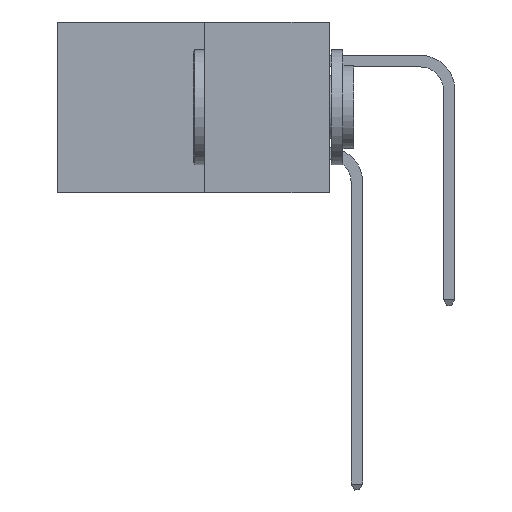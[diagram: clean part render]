
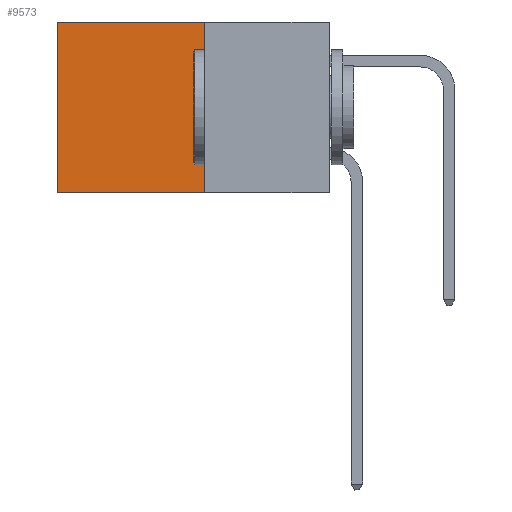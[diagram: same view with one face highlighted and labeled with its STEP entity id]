
A CAD part, left-side view. The second image highlights one B-rep face of the part: STEP entity #9573.
In plain terms, the highlighted planar face has unit normal (-1, 0, 0).
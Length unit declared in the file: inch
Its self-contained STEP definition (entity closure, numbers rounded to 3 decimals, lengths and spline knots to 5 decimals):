
#390 = EDGE_LOOP ( 'NONE', ( #5963, #9810, #3306, #10971 ) ) ;
#1177 = AXIS2_PLACEMENT_3D ( 'NONE', #8500, #1960, #11055 ) ;
#1795 = EDGE_CURVE ( 'NONE', #16024, #11782, #13742, .T. ) ;
#1960 = DIRECTION ( 'NONE',  ( 1., 0., 0. ) ) ;
#1963 = FACE_OUTER_BOUND ( 'NONE', #390, .T. ) ;
#2364 = CARTESIAN_POINT ( 'NONE',  ( 0.277, 0.27, -0.37 ) ) ;
#2398 = DIRECTION ( 'NONE',  ( 0., 1., 0. ) ) ;
#3306 = ORIENTED_EDGE ( 'NONE', *, *, #1795, .F. ) ;
#3392 = DIRECTION ( 'NONE',  ( 0., 0., -1. ) ) ;
#4226 = DIRECTION ( 'NONE',  ( 0., 0., -1. ) ) ;
#4385 = VECTOR ( 'NONE', #2398, 39.37008 ) ;
#4651 = CARTESIAN_POINT ( 'NONE',  ( 0.277, 0.27, -0.37 ) ) ;
#4692 = VECTOR ( 'NONE', #3392, 39.37008 ) ;
#4784 = LINE ( 'NONE', #2364, #4385 ) ;
#4790 = CARTESIAN_POINT ( 'NONE',  ( 0.277, 0.59, -0.37 ) ) ;
#4817 = DIRECTION ( 'NONE',  ( 0., 1., 0. ) ) ;
#5425 = CARTESIAN_POINT ( 'NONE',  ( 0.277, 0.27, -0.37 ) ) ;
#5963 = ORIENTED_EDGE ( 'NONE', *, *, #9622, .T. ) ;
#6109 = CARTESIAN_POINT ( 'NONE',  ( 0.277, 0.27, 0. ) ) ;
#6178 = EDGE_CURVE ( 'NONE', #11782, #8826, #4784, .T. ) ;
#8098 = LINE ( 'NONE', #6109, #14401 ) ;
#8128 = LINE ( 'NONE', #8565, #4692 ) ;
#8500 = CARTESIAN_POINT ( 'NONE',  ( 0.277, 0.27, -0.37 ) ) ;
#8565 = CARTESIAN_POINT ( 'NONE',  ( 0.277, 0.59, -0.37 ) ) ;
#8826 = VERTEX_POINT ( 'NONE', #4790 ) ;
#9573 = ADVANCED_FACE ( 'NONE', ( #1963 ), #15888, .F. ) ;
#9603 = CARTESIAN_POINT ( 'NONE',  ( 0.277, 0.59, 0. ) ) ;
#9622 = EDGE_CURVE ( 'NONE', #15442, #8826, #8128, .T. ) ;
#9810 = ORIENTED_EDGE ( 'NONE', *, *, #6178, .F. ) ;
#10397 = VECTOR ( 'NONE', #4226, 39.37008 ) ;
#10971 = ORIENTED_EDGE ( 'NONE', *, *, #11932, .T. ) ;
#11055 = DIRECTION ( 'NONE',  ( 0., 0., -1. ) ) ;
#11782 = VERTEX_POINT ( 'NONE', #4651 ) ;
#11932 = EDGE_CURVE ( 'NONE', #16024, #15442, #8098, .T. ) ;
#13742 = LINE ( 'NONE', #5425, #10397 ) ;
#14401 = VECTOR ( 'NONE', #4817, 39.37008 ) ;
#14439 = CARTESIAN_POINT ( 'NONE',  ( 0.277, 0.27, 0. ) ) ;
#15442 = VERTEX_POINT ( 'NONE', #9603 ) ;
#15888 = PLANE ( 'NONE',  #1177 ) ;
#16024 = VERTEX_POINT ( 'NONE', #14439 ) ;
